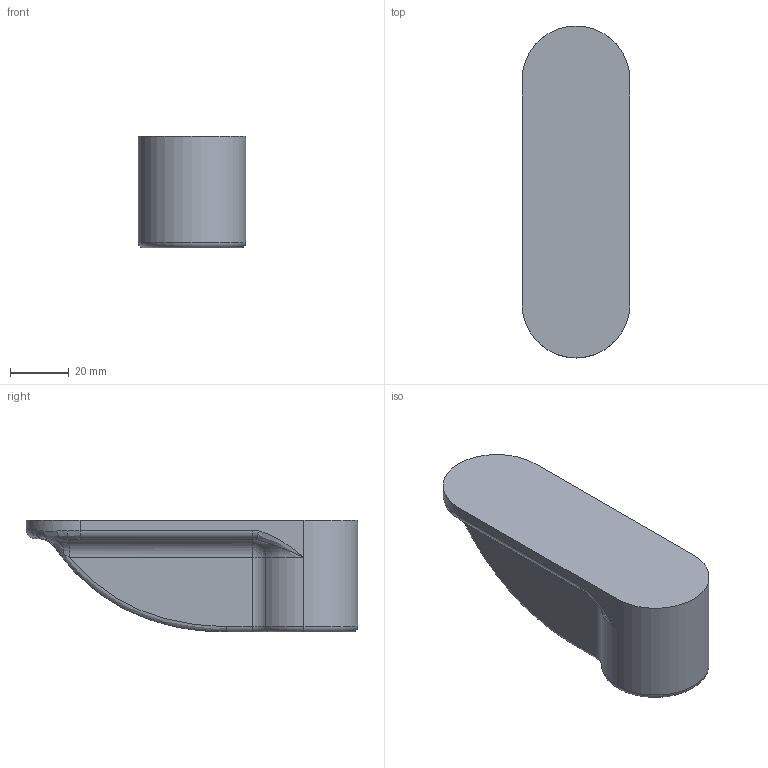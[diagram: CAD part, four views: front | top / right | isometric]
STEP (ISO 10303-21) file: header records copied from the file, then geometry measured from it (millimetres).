
FILE_DESCRIPTION (( 'STEP AP214' ), '1' );
FILE_NAME ('Minimalist Stock.STEP', '2014-02-08T04:55:07', ( 'elpi' ), ( '' ), 'SwSTEP 2.0', 'SolidWorks 2013', '' );
FILE_SCHEMA (( 'AUTOMOTIVE_DESIGN' ));
Length unit declared in the file: inch
Products named in the file (1): Minimalist Stock
Bounding box: 36.7 x 112.9 x 38.1 mm (x, y, z)
Volume: 56492.2 mm3; surface area: 20460.4 mm2
Topology: 1 solids, 1 shells, 106 faces, 242 edges, 134 vertices
Faces by surface type: bspline 37, cylinder 31, torus 19, plane 15, sphere 4
Entity records: 4188 total; most frequent: CARTESIAN_POINT 1991, ORIENTED_EDGE 476, DIRECTION 433, EDGE_CURVE 238, AXIS2_PLACEMENT_3D 188, VERTEX_POINT 134, CIRCLE 118, EDGE_LOOP 108
